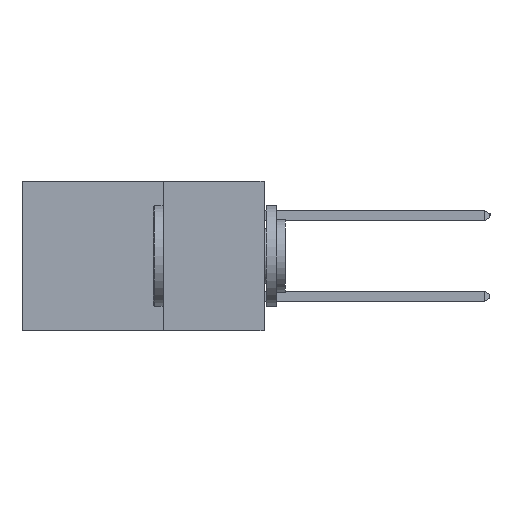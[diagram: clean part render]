
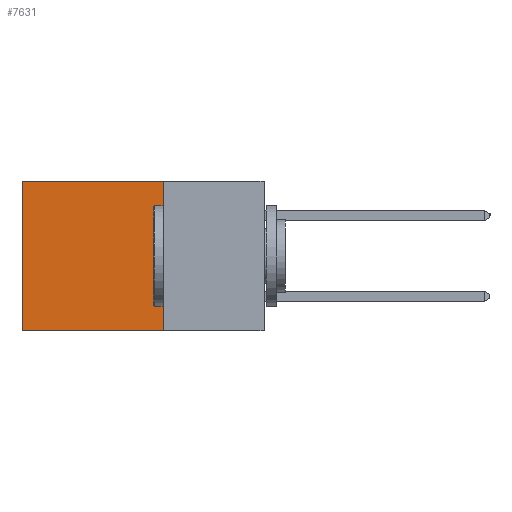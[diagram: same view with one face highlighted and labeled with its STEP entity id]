
A CAD part, left-side view. The second image highlights one B-rep face of the part: STEP entity #7631.
In plain terms, the highlighted planar face has unit normal (-1, 0, 0).
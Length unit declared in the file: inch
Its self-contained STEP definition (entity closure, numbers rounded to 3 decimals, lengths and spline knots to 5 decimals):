
#324 = EDGE_LOOP ( 'NONE', ( #6825, #10565, #11807, #16422 ) ) ;
#485 = CARTESIAN_POINT ( 'NONE',  ( 0.2615, 0.6, 0. ) ) ;
#510 = CARTESIAN_POINT ( 'NONE',  ( 0.2615, 0.25, -0.37 ) ) ;
#1561 = DIRECTION ( 'NONE',  ( 0., 0., -1. ) ) ;
#2084 = CARTESIAN_POINT ( 'NONE',  ( 0.2615, 0.25, -0.37 ) ) ;
#2547 = VECTOR ( 'NONE', #10788, 39.37008 ) ;
#3261 = LINE ( 'NONE', #2084, #6454 ) ;
#4409 = CARTESIAN_POINT ( 'NONE',  ( 0.2615, 0.25, -0.37 ) ) ;
#4518 = EDGE_CURVE ( 'NONE', #11943, #16281, #3261, .T. ) ;
#6052 = DIRECTION ( 'NONE',  ( 1., 0., 0. ) ) ;
#6454 = VECTOR ( 'NONE', #10063, 39.37008 ) ;
#6825 = ORIENTED_EDGE ( 'NONE', *, *, #7051, .T. ) ;
#7051 = EDGE_CURVE ( 'NONE', #14564, #12539, #10069, .T. ) ;
#7408 = PLANE ( 'NONE',  #16095 ) ;
#7631 = ADVANCED_FACE ( 'NONE', ( #8949 ), #7408, .F. ) ;
#8949 = FACE_OUTER_BOUND ( 'NONE', #324, .T. ) ;
#9880 = LINE ( 'NONE', #11064, #10358 ) ;
#9901 = CARTESIAN_POINT ( 'NONE',  ( 0.2615, 0.6, -0.37 ) ) ;
#10020 = EDGE_CURVE ( 'NONE', #16281, #12539, #9880, .T. ) ;
#10063 = DIRECTION ( 'NONE',  ( 0., 0., -1. ) ) ;
#10069 = LINE ( 'NONE', #9901, #15801 ) ;
#10302 = CARTESIAN_POINT ( 'NONE',  ( 0.2615, 0.25, 0. ) ) ;
#10358 = VECTOR ( 'NONE', #12614, 39.37008 ) ;
#10565 = ORIENTED_EDGE ( 'NONE', *, *, #10020, .F. ) ;
#10788 = DIRECTION ( 'NONE',  ( 0., 1., 0. ) ) ;
#10877 = CARTESIAN_POINT ( 'NONE',  ( 0.2615, 0.6, -0.37 ) ) ;
#11064 = CARTESIAN_POINT ( 'NONE',  ( 0.2615, 0.25, -0.37 ) ) ;
#11807 = ORIENTED_EDGE ( 'NONE', *, *, #4518, .F. ) ;
#11943 = VERTEX_POINT ( 'NONE', #10302 ) ;
#12539 = VERTEX_POINT ( 'NONE', #10877 ) ;
#12614 = DIRECTION ( 'NONE',  ( 0., 1., 0. ) ) ;
#13534 = LINE ( 'NONE', #16340, #2547 ) ;
#13813 = EDGE_CURVE ( 'NONE', #11943, #14564, #13534, .T. ) ;
#14517 = DIRECTION ( 'NONE',  ( 0., 0., -1. ) ) ;
#14564 = VERTEX_POINT ( 'NONE', #485 ) ;
#15801 = VECTOR ( 'NONE', #1561, 39.37008 ) ;
#16095 = AXIS2_PLACEMENT_3D ( 'NONE', #510, #6052, #14517 ) ;
#16281 = VERTEX_POINT ( 'NONE', #4409 ) ;
#16340 = CARTESIAN_POINT ( 'NONE',  ( 0.2615, 0.25, 0. ) ) ;
#16422 = ORIENTED_EDGE ( 'NONE', *, *, #13813, .T. ) ;
